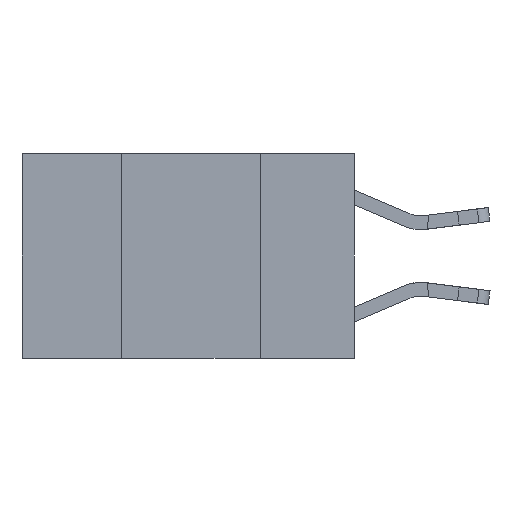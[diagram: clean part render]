
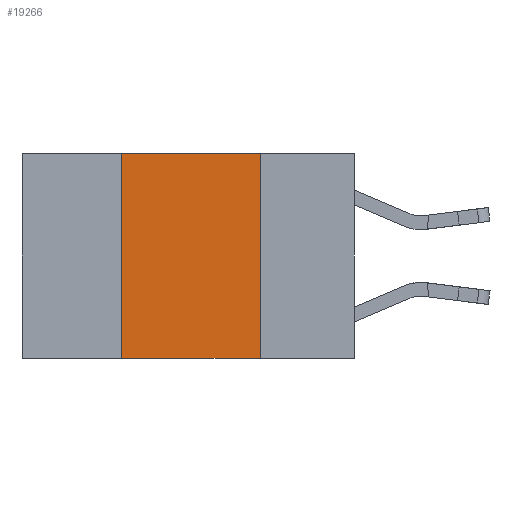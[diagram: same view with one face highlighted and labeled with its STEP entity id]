
A CAD part, left-side view. The second image highlights one B-rep face of the part: STEP entity #19266.
In plain terms, the highlighted planar face has unit normal (-1, 0, 0).
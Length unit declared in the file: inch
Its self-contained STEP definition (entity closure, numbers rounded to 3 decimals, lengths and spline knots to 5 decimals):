
#708 = CARTESIAN_POINT ( 'NONE',  ( 0., 0.42, -0.37 ) ) ;
#1382 = VECTOR ( 'NONE', #8732, 39.37008 ) ;
#2068 = VECTOR ( 'NONE', #6697, 39.37008 ) ;
#3373 = VERTEX_POINT ( 'NONE', #8819 ) ;
#3446 = CARTESIAN_POINT ( 'NONE',  ( 0., 0.17, 0. ) ) ;
#3676 = VECTOR ( 'NONE', #22152, 39.37008 ) ;
#3817 = PLANE ( 'NONE',  #14620 ) ;
#4053 = VERTEX_POINT ( 'NONE', #22805 ) ;
#5878 = CARTESIAN_POINT ( 'NONE',  ( 0., 0.6, 0. ) ) ;
#5927 = DIRECTION ( 'NONE',  ( 1., 0., 0. ) ) ;
#6697 = DIRECTION ( 'NONE',  ( 0., -1., 0. ) ) ;
#6934 = EDGE_LOOP ( 'NONE', ( #10293, #15713, #10193, #15618 ) ) ;
#8732 = DIRECTION ( 'NONE',  ( 0., 0., 1. ) ) ;
#8819 = CARTESIAN_POINT ( 'NONE',  ( 0., 0.17, 0. ) ) ;
#10193 = ORIENTED_EDGE ( 'NONE', *, *, #24380, .F. ) ;
#10293 = ORIENTED_EDGE ( 'NONE', *, *, #19834, .F. ) ;
#10716 = VERTEX_POINT ( 'NONE', #20570 ) ;
#13056 = LINE ( 'NONE', #20970, #2068 ) ;
#13280 = EDGE_CURVE ( 'NONE', #4053, #3373, #14655, .T. ) ;
#13598 = EDGE_CURVE ( 'NONE', #18349, #10716, #13056, .T. ) ;
#14620 = AXIS2_PLACEMENT_3D ( 'NONE', #16127, #5927, #20137 ) ;
#14655 = LINE ( 'NONE', #5878, #3676 ) ;
#15618 = ORIENTED_EDGE ( 'NONE', *, *, #13598, .T. ) ;
#15713 = ORIENTED_EDGE ( 'NONE', *, *, #13280, .F. ) ;
#15850 = LINE ( 'NONE', #20868, #1382 ) ;
#16127 = CARTESIAN_POINT ( 'NONE',  ( 0., 0.6, 0. ) ) ;
#18349 = VERTEX_POINT ( 'NONE', #708 ) ;
#19266 = ADVANCED_FACE ( 'NONE', ( #26249 ), #3817, .F. ) ;
#19766 = DIRECTION ( 'NONE',  ( 0., 0., -1. ) ) ;
#19834 = EDGE_CURVE ( 'NONE', #3373, #10716, #23736, .T. ) ;
#20137 = DIRECTION ( 'NONE',  ( 0., 0., -1. ) ) ;
#20570 = CARTESIAN_POINT ( 'NONE',  ( 0., 0.17, -0.37 ) ) ;
#20868 = CARTESIAN_POINT ( 'NONE',  ( 0., 0.42, 0. ) ) ;
#20970 = CARTESIAN_POINT ( 'NONE',  ( 0., 0.6, -0.37 ) ) ;
#22152 = DIRECTION ( 'NONE',  ( 0., -1., 0. ) ) ;
#22805 = CARTESIAN_POINT ( 'NONE',  ( 0., 0.42, 0. ) ) ;
#23116 = VECTOR ( 'NONE', #19766, 39.37008 ) ;
#23736 = LINE ( 'NONE', #3446, #23116 ) ;
#24380 = EDGE_CURVE ( 'NONE', #18349, #4053, #15850, .T. ) ;
#26249 = FACE_OUTER_BOUND ( 'NONE', #6934, .T. ) ;
